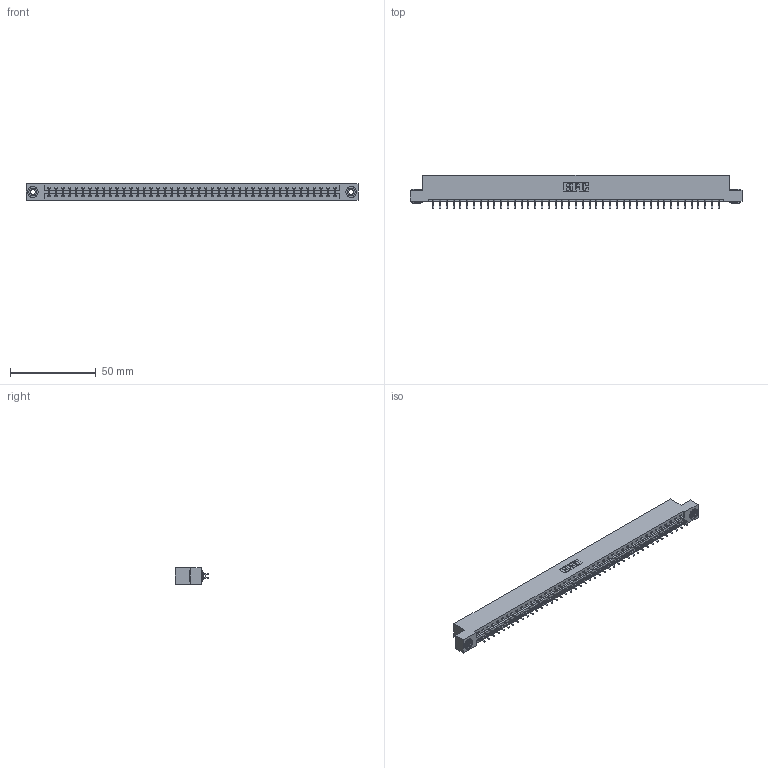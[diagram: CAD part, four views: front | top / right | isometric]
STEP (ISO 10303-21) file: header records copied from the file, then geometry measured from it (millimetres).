
FILE_DESCRIPTION (( 'STEP AP203' ), '1' );
FILE_NAME ('337-086-556-203.STEP', '2019-10-10T15:19:45', ( '' ), ( '' ), 'SwSTEP 2.0', 'SolidWorks 2016', '' );
FILE_SCHEMA (( 'CONFIG_CONTROL_DESIGN' ));
Length unit declared in the file: inch
Products named in the file (4): 345-292-001_556 Tail; 345-250-002_345-250-002-102; 337-086-556-203; 337 Part_Flush Mounting Lugs - 0.156 Dia-TH
Assembly tree (89 placements, depth 2):
  337-086-556-203
    337 Part_Flush Mounting Lugs - 0.156 Dia-TH
    345-292-001_556 Tail  x86
    345-250-002_345-250-002-102  x2
Bounding box: 193.4 x 19.57 x 9.4 mm (x, y, z)
Volume: 20410.9 mm3; surface area: 23217.9 mm2
Topology: 89 solids, 89 shells, 5312 faces, 15781 edges, 10402 vertices
Faces by surface type: plane 3692, cylinder 1612, cone 8
Entity records: 34080 total; most frequent: CARTESIAN_POINT 5729, ORIENTED_EDGE 5646, DIRECTION 4893, EDGE_CURVE 2823, VECTOR 2663, LINE 2663, VERTEX_POINT 1878, AXIS2_PLACEMENT_3D 1115
